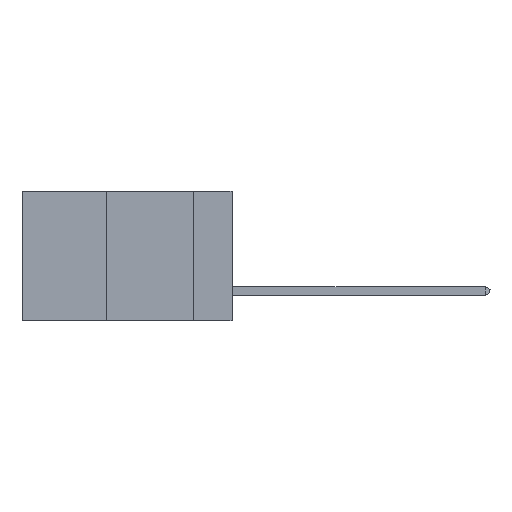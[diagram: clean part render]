
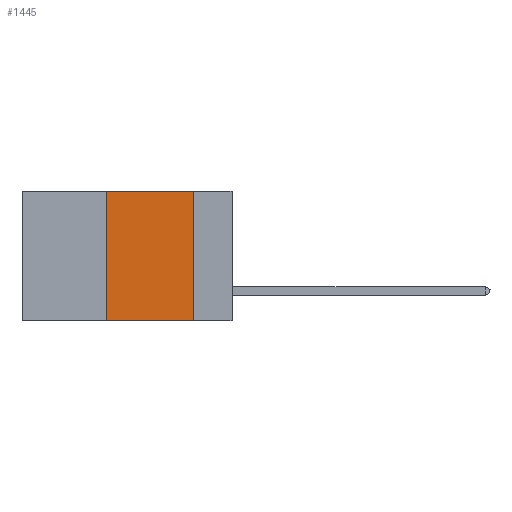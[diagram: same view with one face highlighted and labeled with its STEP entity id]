
A CAD part, left-side view. The second image highlights one B-rep face of the part: STEP entity #1445.
In plain terms, the highlighted planar face has unit normal (-1, 0, 0).
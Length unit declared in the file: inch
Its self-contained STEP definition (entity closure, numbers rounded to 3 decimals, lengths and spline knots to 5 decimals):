
#354 = ORIENTED_EDGE ( 'NONE', *, *, #2885, .F. ) ;
#1445 = ADVANCED_FACE ( 'NONE', ( #39004 ), #38877, .F. ) ;
#1744 = DIRECTION ( 'NONE',  ( 0., 0., -1. ) ) ;
#2300 = LINE ( 'NONE', #12501, #15509 ) ;
#2885 = EDGE_CURVE ( 'NONE', #32026, #42004, #2300, .T. ) ;
#3058 = DIRECTION ( 'NONE',  ( 0., -1., 0. ) ) ;
#4180 = CARTESIAN_POINT ( 'NONE',  ( 0., 0.36, 0. ) ) ;
#5474 = LINE ( 'NONE', #4180, #12356 ) ;
#6504 = ORIENTED_EDGE ( 'NONE', *, *, #41160, .F. ) ;
#7304 = DIRECTION ( 'NONE',  ( 0., 0., -1. ) ) ;
#8429 = LINE ( 'NONE', #10987, #41769 ) ;
#8468 = CARTESIAN_POINT ( 'NONE',  ( 0., 0.11, 0. ) ) ;
#8667 = EDGE_CURVE ( 'NONE', #43076, #30829, #42092, .T. ) ;
#10987 = CARTESIAN_POINT ( 'NONE',  ( 0., 0.11, 0. ) ) ;
#11928 = DIRECTION ( 'NONE',  ( 1., 0., 0. ) ) ;
#12081 = CARTESIAN_POINT ( 'NONE',  ( 0., 0.6, 0. ) ) ;
#12356 = VECTOR ( 'NONE', #21972, 39.37008 ) ;
#12501 = CARTESIAN_POINT ( 'NONE',  ( 0., 0.6, 0. ) ) ;
#12685 = CARTESIAN_POINT ( 'NONE',  ( 0., 0.36, 0. ) ) ;
#13347 = CARTESIAN_POINT ( 'NONE',  ( 0., 0.36, -0.37 ) ) ;
#15509 = VECTOR ( 'NONE', #23317, 39.37008 ) ;
#21972 = DIRECTION ( 'NONE',  ( 0., 0., 1. ) ) ;
#23306 = AXIS2_PLACEMENT_3D ( 'NONE', #12081, #11928, #1744 ) ;
#23317 = DIRECTION ( 'NONE',  ( 0., -1., 0. ) ) ;
#26365 = EDGE_CURVE ( 'NONE', #42004, #30829, #8429, .T. ) ;
#29285 = EDGE_LOOP ( 'NONE', ( #32024, #354, #6504, #32525 ) ) ;
#30829 = VERTEX_POINT ( 'NONE', #38964 ) ;
#32024 = ORIENTED_EDGE ( 'NONE', *, *, #26365, .F. ) ;
#32026 = VERTEX_POINT ( 'NONE', #12685 ) ;
#32525 = ORIENTED_EDGE ( 'NONE', *, *, #8667, .T. ) ;
#38872 = VECTOR ( 'NONE', #3058, 39.37008 ) ;
#38877 = PLANE ( 'NONE',  #23306 ) ;
#38964 = CARTESIAN_POINT ( 'NONE',  ( 0., 0.11, -0.37 ) ) ;
#39004 = FACE_OUTER_BOUND ( 'NONE', #29285, .T. ) ;
#40645 = CARTESIAN_POINT ( 'NONE',  ( 0., 0.6, -0.37 ) ) ;
#41160 = EDGE_CURVE ( 'NONE', #43076, #32026, #5474, .T. ) ;
#41769 = VECTOR ( 'NONE', #7304, 39.37008 ) ;
#42004 = VERTEX_POINT ( 'NONE', #8468 ) ;
#42092 = LINE ( 'NONE', #40645, #38872 ) ;
#43076 = VERTEX_POINT ( 'NONE', #13347 ) ;
